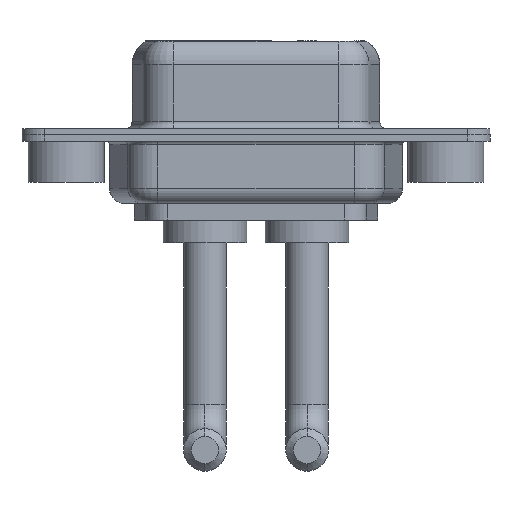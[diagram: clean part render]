
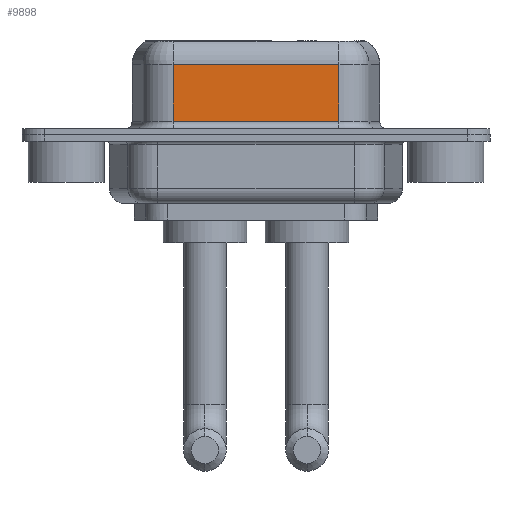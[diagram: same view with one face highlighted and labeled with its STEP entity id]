
A CAD part, front view. The second image highlights one B-rep face of the part: STEP entity #9898.
In plain terms, the highlighted planar face has unit normal (0, -1, 0).
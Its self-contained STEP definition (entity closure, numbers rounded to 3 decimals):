
#51 = VERTEX_POINT ( 'NONE', #12495 ) ;
#683 = LINE ( 'NONE', #3694, #10993 ) ;
#1061 = VERTEX_POINT ( 'NONE', #8343 ) ;
#1395 = ORIENTED_EDGE ( 'NONE', *, *, #8925, .F. ) ;
#2542 = VECTOR ( 'NONE', #5803, 1000. ) ;
#2689 = EDGE_CURVE ( 'NONE', #51, #1061, #13228, .T. ) ;
#2793 = VERTEX_POINT ( 'NONE', #4601 ) ;
#3190 = CARTESIAN_POINT ( 'NONE',  ( 7.038, -3.95, 6.4 ) ) ;
#3371 = ORIENTED_EDGE ( 'NONE', *, *, #2689, .T. ) ;
#3460 = LINE ( 'NONE', #8775, #2542 ) ;
#3694 = CARTESIAN_POINT ( 'NONE',  ( 17.962, -3.95, 0.9 ) ) ;
#4601 = CARTESIAN_POINT ( 'NONE',  ( 17.962, -3.95, 0.9 ) ) ;
#4647 = DIRECTION ( 'NONE',  ( 0., 1., 0. ) ) ;
#4666 = DIRECTION ( 'NONE',  ( -1., 0., 0. ) ) ;
#5243 = VECTOR ( 'NONE', #9512, 1000. ) ;
#5803 = DIRECTION ( 'NONE',  ( 0., 0., -1. ) ) ;
#5932 = EDGE_CURVE ( 'NONE', #12350, #51, #7002, .T. ) ;
#6435 = AXIS2_PLACEMENT_3D ( 'NONE', #7523, #4647, #9557 ) ;
#6587 = VECTOR ( 'NONE', #4666, 1000. ) ;
#6659 = FACE_OUTER_BOUND ( 'NONE', #13116, .T. ) ;
#7002 = LINE ( 'NONE', #12119, #6587 ) ;
#7523 = CARTESIAN_POINT ( 'NONE',  ( 17.962, -3.95, 6.4 ) ) ;
#7983 = ORIENTED_EDGE ( 'NONE', *, *, #12129, .T. ) ;
#8343 = CARTESIAN_POINT ( 'NONE',  ( 7.038, -3.95, 0.9 ) ) ;
#8356 = ORIENTED_EDGE ( 'NONE', *, *, #5932, .T. ) ;
#8520 = CARTESIAN_POINT ( 'NONE',  ( 17.962, -3.95, 4.65 ) ) ;
#8775 = CARTESIAN_POINT ( 'NONE',  ( 17.962, -3.95, 6.4 ) ) ;
#8925 = EDGE_CURVE ( 'NONE', #12350, #2793, #3460, .T. ) ;
#9512 = DIRECTION ( 'NONE',  ( 0., 0., -1. ) ) ;
#9557 = DIRECTION ( 'NONE',  ( -1., 0., 0. ) ) ;
#9898 = ADVANCED_FACE ( 'NONE', ( #6659 ), #10565, .F. ) ;
#10565 = PLANE ( 'NONE',  #6435 ) ;
#10993 = VECTOR ( 'NONE', #11217, 1000. ) ;
#11217 = DIRECTION ( 'NONE',  ( 1., 0., 0. ) ) ;
#12119 = CARTESIAN_POINT ( 'NONE',  ( 17.962, -3.95, 4.65 ) ) ;
#12129 = EDGE_CURVE ( 'NONE', #1061, #2793, #683, .T. ) ;
#12350 = VERTEX_POINT ( 'NONE', #8520 ) ;
#12495 = CARTESIAN_POINT ( 'NONE',  ( 7.038, -3.95, 4.65 ) ) ;
#13116 = EDGE_LOOP ( 'NONE', ( #1395, #8356, #3371, #7983 ) ) ;
#13228 = LINE ( 'NONE', #3190, #5243 ) ;
